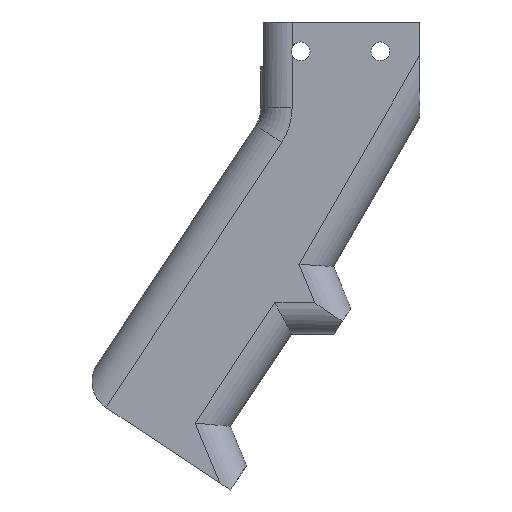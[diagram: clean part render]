
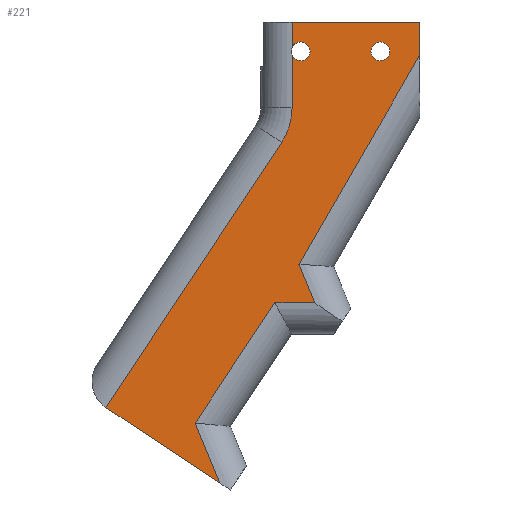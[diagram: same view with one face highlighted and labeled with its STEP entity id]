
A CAD part, front view. The second image highlights one B-rep face of the part: STEP entity #221.
In plain terms, the highlighted planar face has unit normal (0, -1, 0).
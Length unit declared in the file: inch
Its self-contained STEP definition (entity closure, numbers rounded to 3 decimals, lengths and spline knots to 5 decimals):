
#6 = DIRECTION ( 'NONE',  ( -0.833, 0., 0.553 ) ) ;
#13 = DIRECTION ( 'NONE',  ( 0., -1., 0. ) ) ;
#18 = VERTEX_POINT ( 'NONE', #822 ) ;
#72 = VERTEX_POINT ( 'NONE', #222 ) ;
#77 = VECTOR ( 'NONE', #909, 39.37008 ) ;
#98 = ORIENTED_EDGE ( 'NONE', *, *, #813, .F. ) ;
#104 = DIRECTION ( 'NONE',  ( -0.553, 0., -0.833 ) ) ;
#122 = EDGE_CURVE ( 'NONE', #480, #299, #1389, .T. ) ;
#137 = CIRCLE ( 'NONE', #943, 0.15 ) ;
#156 = CARTESIAN_POINT ( 'NONE',  ( 0.61048, 0., -3.16297 ) ) ;
#177 = CARTESIAN_POINT ( 'NONE',  ( 0.5, 0., 0.30995 ) ) ;
#190 = EDGE_CURVE ( 'NONE', #72, #923, #1297, .T. ) ;
#207 = CARTESIAN_POINT ( 'NONE',  ( 0.5, 0., -0.80663 ) ) ;
#210 = CARTESIAN_POINT ( 'NONE',  ( 1.89657, 0., -1.25728 ) ) ;
#221 = ADVANCED_FACE ( 'NONE', ( #392, #1350 ), #353, .T. ) ;
#222 = CARTESIAN_POINT ( 'NONE',  ( 1.9125, 0., 0.4 ) ) ;
#242 = AXIS2_PLACEMENT_3D ( 'NONE', #616, #1074, #379 ) ;
#251 = VECTOR ( 'NONE', #853, 39.37008 ) ;
#256 = CARTESIAN_POINT ( 'NONE',  ( 2.55, 0., 0.72 ) ) ;
#258 = CARTESIAN_POINT ( 'NONE',  ( 0.6375, 0., 0.25 ) ) ;
#268 = EDGE_CURVE ( 'NONE', #1265, #402, #776, .T. ) ;
#275 = CARTESIAN_POINT ( 'NONE',  ( 0.6375, 0., 0.1 ) ) ;
#295 = CARTESIAN_POINT ( 'NONE',  ( -1.05313, 0., -5.70683 ) ) ;
#299 = VERTEX_POINT ( 'NONE', #156 ) ;
#313 = DIRECTION ( 'NONE',  ( 0., 0., -1. ) ) ;
#325 = VECTOR ( 'NONE', #544, 39.37008 ) ;
#328 = ORIENTED_EDGE ( 'NONE', *, *, #652, .T. ) ;
#342 = CARTESIAN_POINT ( 'NONE',  ( 2.55, 0., -0.80663 ) ) ;
#353 = PLANE ( 'NONE',  #619 ) ;
#360 = CIRCLE ( 'NONE', #1273, 0.15 ) ;
#371 = ORIENTED_EDGE ( 'NONE', *, *, #1411, .T. ) ;
#379 = DIRECTION ( 'NONE',  ( 0., 0., -1. ) ) ;
#392 = FACE_BOUND ( 'NONE', #1150, .T. ) ;
#401 = CARTESIAN_POINT ( 'NONE',  ( 0.33349, 0., -1.20849 ) ) ;
#402 = VERTEX_POINT ( 'NONE', #177 ) ;
#438 = EDGE_CURVE ( 'NONE', #923, #72, #523, .T. ) ;
#441 = ORIENTED_EDGE ( 'NONE', *, *, #438, .F. ) ;
#445 = LINE ( 'NONE', #1162, #251 ) ;
#447 = LINE ( 'NONE', #207, #1042 ) ;
#460 = DIRECTION ( 'NONE',  ( -0.379, 0., 0.925 ) ) ;
#469 = DIRECTION ( 'NONE',  ( 0., -1., 0. ) ) ;
#476 = CARTESIAN_POINT ( 'NONE',  ( 0.2231, 0., -3.78167 ) ) ;
#477 = DIRECTION ( 'NONE',  ( 0., 0., -1. ) ) ;
#480 = VERTEX_POINT ( 'NONE', #1114 ) ;
#483 = CARTESIAN_POINT ( 'NONE',  ( 1.9125, 0., 0.25 ) ) ;
#491 = CARTESIAN_POINT ( 'NONE',  ( 0., 0., 0. ) ) ;
#500 = ORIENTED_EDGE ( 'NONE', *, *, #268, .T. ) ;
#505 = VECTOR ( 'NONE', #1146, 39.37008 ) ;
#523 = CIRCLE ( 'NONE', #675, 0.15 ) ;
#530 = CARTESIAN_POINT ( 'NONE',  ( 0.6375, 0., 0.25 ) ) ;
#533 = ORIENTED_EDGE ( 'NONE', *, *, #1119, .F. ) ;
#539 = VECTOR ( 'NONE', #104, 39.37008 ) ;
#540 = EDGE_CURVE ( 'NONE', #1343, #480, #1313, .T. ) ;
#543 = VERTEX_POINT ( 'NONE', #918 ) ;
#544 = DIRECTION ( 'NONE',  ( 1., 0., 0. ) ) ;
#549 = ORIENTED_EDGE ( 'NONE', *, *, #122, .T. ) ;
#567 = CARTESIAN_POINT ( 'NONE',  ( 0.6375, 0., 0.25 ) ) ;
#574 = EDGE_CURVE ( 'NONE', #543, #18, #447, .T. ) ;
#579 = CARTESIAN_POINT ( 'NONE',  ( -0.58626, 0., -0.24004 ) ) ;
#580 = EDGE_CURVE ( 'NONE', #1440, #1415, #1470, .T. ) ;
#582 = CARTESIAN_POINT ( 'NONE',  ( -0.65972, 0., -6.66769 ) ) ;
#616 = CARTESIAN_POINT ( 'NONE',  ( -0.5, 0., -0.65595 ) ) ;
#619 = AXIS2_PLACEMENT_3D ( 'NONE', #491, #1421, #477 ) ;
#621 = LINE ( 'NONE', #210, #77 ) ;
#627 = VERTEX_POINT ( 'NONE', #582 ) ;
#633 = VECTOR ( 'NONE', #1148, 39.37008 ) ;
#647 = DIRECTION ( 'NONE',  ( 0., 0., -1. ) ) ;
#652 = EDGE_CURVE ( 'NONE', #627, #1001, #1436, .T. ) ;
#654 = VECTOR ( 'NONE', #702, 39.37008 ) ;
#671 = ORIENTED_EDGE ( 'NONE', *, *, #818, .F. ) ;
#675 = AXIS2_PLACEMENT_3D ( 'NONE', #1243, #1232, #1356 ) ;
#696 = CARTESIAN_POINT ( 'NONE',  ( -2.90304, 0., -1.1886 ) ) ;
#702 = DIRECTION ( 'NONE',  ( -0.379, 0., 0.925 ) ) ;
#720 = AXIS2_PLACEMENT_3D ( 'NONE', #258, #1072, #737 ) ;
#737 = DIRECTION ( 'NONE',  ( 0., 0., -1. ) ) ;
#770 = ORIENTED_EDGE ( 'NONE', *, *, #1477, .F. ) ;
#775 = CARTESIAN_POINT ( 'NONE',  ( -2.90063, 0., -5.18215 ) ) ;
#776 = LINE ( 'NONE', #1427, #1242 ) ;
#781 = VERTEX_POINT ( 'NONE', #256 ) ;
#783 = ORIENTED_EDGE ( 'NONE', *, *, #540, .T. ) ;
#805 = AXIS2_PLACEMENT_3D ( 'NONE', #483, #469, #954 ) ;
#813 = EDGE_CURVE ( 'NONE', #872, #1431, #1345, .T. ) ;
#818 = EDGE_CURVE ( 'NONE', #1440, #18, #1039, .T. ) ;
#819 = LINE ( 'NONE', #775, #1021 ) ;
#822 = CARTESIAN_POINT ( 'NONE',  ( 0.5, 0., -0.65595 ) ) ;
#827 = CARTESIAN_POINT ( 'NONE',  ( 0.5, 0., 0.72 ) ) ;
#853 = DIRECTION ( 'NONE',  ( 0.5, 0., 0.866 ) ) ;
#872 = VERTEX_POINT ( 'NONE', #275 ) ;
#884 = DIRECTION ( 'NONE',  ( 0., -1., 0. ) ) ;
#903 = CARTESIAN_POINT ( 'NONE',  ( 2.55, 0., 0.19251 ) ) ;
#904 = ORIENTED_EDGE ( 'NONE', *, *, #574, .T. ) ;
#909 = DIRECTION ( 'NONE',  ( 0.553, 0., 0.833 ) ) ;
#916 = EDGE_LOOP ( 'NONE', ( #1339, #328, #371, #783, #549, #1286, #1115, #533, #500, #770, #98, #1016, #904, #671, #970 ) ) ;
#918 = CARTESIAN_POINT ( 'NONE',  ( 0.5, 0., 0.19005 ) ) ;
#923 = VERTEX_POINT ( 'NONE', #1325 ) ;
#943 = AXIS2_PLACEMENT_3D ( 'NONE', #567, #13, #1386 ) ;
#954 = DIRECTION ( 'NONE',  ( 0., 0., -1. ) ) ;
#970 = ORIENTED_EDGE ( 'NONE', *, *, #580, .T. ) ;
#1001 = VERTEX_POINT ( 'NONE', #295 ) ;
#1015 = CARTESIAN_POINT ( 'NONE',  ( 0.78822, 0., -0.52253 ) ) ;
#1016 = ORIENTED_EDGE ( 'NONE', *, *, #1414, .F. ) ;
#1020 = CARTESIAN_POINT ( 'NONE',  ( 0., 0., -3.78167 ) ) ;
#1021 = VECTOR ( 'NONE', #6, 39.37008 ) ;
#1023 = CARTESIAN_POINT ( 'NONE',  ( 0., 0., 0.72 ) ) ;
#1034 = VERTEX_POINT ( 'NONE', #903 ) ;
#1039 = CIRCLE ( 'NONE', #242, 1. ) ;
#1042 = VECTOR ( 'NONE', #313, 39.37008 ) ;
#1072 = DIRECTION ( 'NONE',  ( 0., -1., 0. ) ) ;
#1074 = DIRECTION ( 'NONE',  ( 0., -1., 0. ) ) ;
#1099 = EDGE_CURVE ( 'NONE', #627, #1415, #819, .T. ) ;
#1114 = CARTESIAN_POINT ( 'NONE',  ( 0.8638, 0., -3.78167 ) ) ;
#1115 = ORIENTED_EDGE ( 'NONE', *, *, #1145, .F. ) ;
#1119 = EDGE_CURVE ( 'NONE', #1265, #781, #1405, .T. ) ;
#1145 = EDGE_CURVE ( 'NONE', #781, #1034, #1403, .T. ) ;
#1146 = DIRECTION ( 'NONE',  ( 1., 0., 0. ) ) ;
#1148 = DIRECTION ( 'NONE',  ( 0., 0., -1. ) ) ;
#1150 = EDGE_LOOP ( 'NONE', ( #1166, #441 ) ) ;
#1162 = CARTESIAN_POINT ( 'NONE',  ( 1.82799, 0., -1.05661 ) ) ;
#1166 = ORIENTED_EDGE ( 'NONE', *, *, #190, .F. ) ;
#1232 = DIRECTION ( 'NONE',  ( 0., -1., 0. ) ) ;
#1242 = VECTOR ( 'NONE', #1438, 39.37008 ) ;
#1243 = CARTESIAN_POINT ( 'NONE',  ( 1.9125, 0., 0.25 ) ) ;
#1265 = VERTEX_POINT ( 'NONE', #827 ) ;
#1273 = AXIS2_PLACEMENT_3D ( 'NONE', #530, #884, #647 ) ;
#1278 = VECTOR ( 'NONE', #460, 39.37008 ) ;
#1286 = ORIENTED_EDGE ( 'NONE', *, *, #1362, .T. ) ;
#1297 = CIRCLE ( 'NONE', #805, 0.15 ) ;
#1313 = LINE ( 'NONE', #1020, #325 ) ;
#1325 = CARTESIAN_POINT ( 'NONE',  ( 1.9125, 0., 0.1 ) ) ;
#1339 = ORIENTED_EDGE ( 'NONE', *, *, #1099, .F. ) ;
#1343 = VERTEX_POINT ( 'NONE', #476 ) ;
#1345 = CIRCLE ( 'NONE', #720, 0.15 ) ;
#1349 = CARTESIAN_POINT ( 'NONE',  ( -2.48388, 0., -5.45842 ) ) ;
#1350 = FACE_OUTER_BOUND ( 'NONE', #916, .T. ) ;
#1356 = DIRECTION ( 'NONE',  ( 0., 0., -1. ) ) ;
#1362 = EDGE_CURVE ( 'NONE', #299, #1034, #445, .T. ) ;
#1386 = DIRECTION ( 'NONE',  ( 0., 0., -1. ) ) ;
#1389 = LINE ( 'NONE', #579, #1278 ) ;
#1403 = LINE ( 'NONE', #342, #633 ) ;
#1405 = LINE ( 'NONE', #1023, #505 ) ;
#1411 = EDGE_CURVE ( 'NONE', #1001, #1343, #621, .T. ) ;
#1414 = EDGE_CURVE ( 'NONE', #543, #872, #360, .T. ) ;
#1415 = VERTEX_POINT ( 'NONE', #1349 ) ;
#1421 = DIRECTION ( 'NONE',  ( 0., -1., 0. ) ) ;
#1427 = CARTESIAN_POINT ( 'NONE',  ( 0.5, 0., -0.80663 ) ) ;
#1431 = VERTEX_POINT ( 'NONE', #1460 ) ;
#1436 = LINE ( 'NONE', #696, #654 ) ;
#1438 = DIRECTION ( 'NONE',  ( 0., 0., -1. ) ) ;
#1440 = VERTEX_POINT ( 'NONE', #401 ) ;
#1460 = CARTESIAN_POINT ( 'NONE',  ( 0.6375, 0., 0.4 ) ) ;
#1470 = LINE ( 'NONE', #1015, #539 ) ;
#1477 = EDGE_CURVE ( 'NONE', #1431, #402, #137, .T. ) ;
